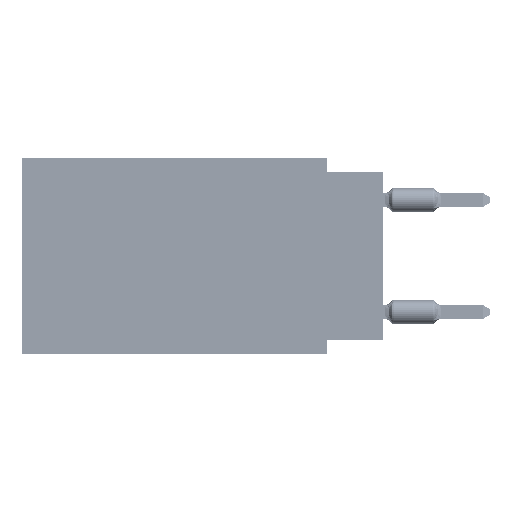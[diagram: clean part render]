
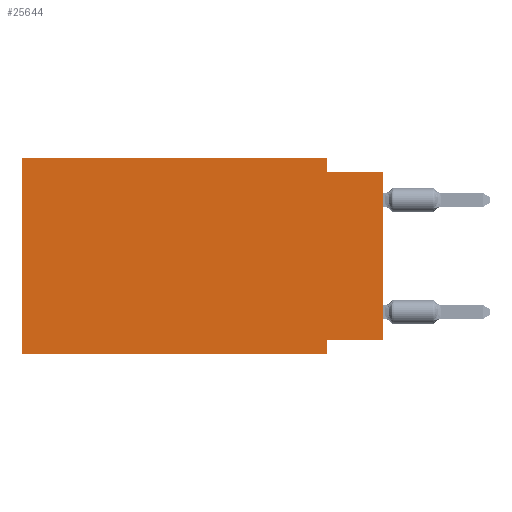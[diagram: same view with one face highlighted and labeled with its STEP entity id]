
A CAD part, left-side view. The second image highlights one B-rep face of the part: STEP entity #25644.
In plain terms, the highlighted planar face has unit normal (-1, 0, 0).
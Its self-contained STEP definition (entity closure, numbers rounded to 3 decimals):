
#2903 = AXIS2_PLACEMENT_3D ( 'NONE', #25191, #89665, #39672 ) ;
#4005 = CARTESIAN_POINT ( 'NONE',  ( 0., 0., -0.635 ) ) ;
#4945 = CARTESIAN_POINT ( 'NONE',  ( 0., 0., 0. ) ) ;
#7699 = CARTESIAN_POINT ( 'NONE',  ( 0., 2.54, -0.635 ) ) ;
#8416 = DIRECTION ( 'NONE',  ( 0., -1., 0. ) ) ;
#8922 = CARTESIAN_POINT ( 'NONE',  ( 0., 16.383, -8.89 ) ) ;
#10558 = VERTEX_POINT ( 'NONE', #29692 ) ;
#10713 = FACE_OUTER_BOUND ( 'NONE', #48097, .T. ) ;
#14119 = VERTEX_POINT ( 'NONE', #87264 ) ;
#14963 = LINE ( 'NONE', #59749, #63827 ) ;
#16705 = ORIENTED_EDGE ( 'NONE', *, *, #35602, .F. ) ;
#18599 = ORIENTED_EDGE ( 'NONE', *, *, #50139, .F. ) ;
#19564 = DIRECTION ( 'NONE',  ( 0., 0., 1. ) ) ;
#20026 = CARTESIAN_POINT ( 'NONE',  ( 0., 16.383, 0. ) ) ;
#20128 = VECTOR ( 'NONE', #69852, 1000. ) ;
#20346 = LINE ( 'NONE', #4005, #20128 ) ;
#20501 = EDGE_CURVE ( 'NONE', #47222, #37222, #57631, .T. ) ;
#20869 = VECTOR ( 'NONE', #86489, 1000. ) ;
#22082 = EDGE_CURVE ( 'NONE', #10558, #37222, #43518, .T. ) ;
#22592 = DIRECTION ( 'NONE',  ( 0., 0., -1. ) ) ;
#25191 = CARTESIAN_POINT ( 'NONE',  ( 0., 16.383, 0. ) ) ;
#25644 = ADVANCED_FACE ( 'NONE', ( #10713 ), #89194, .F. ) ;
#27021 = LINE ( 'NONE', #20026, #58323 ) ;
#28350 = ORIENTED_EDGE ( 'NONE', *, *, #22082, .T. ) ;
#28411 = ORIENTED_EDGE ( 'NONE', *, *, #61844, .T. ) ;
#28534 = VECTOR ( 'NONE', #33438, 1000. ) ;
#29692 = CARTESIAN_POINT ( 'NONE',  ( 0., 16.383, -8.89 ) ) ;
#30540 = LINE ( 'NONE', #59047, #42568 ) ;
#31368 = CARTESIAN_POINT ( 'NONE',  ( 0., 16.383, 0. ) ) ;
#32716 = ORIENTED_EDGE ( 'NONE', *, *, #20501, .F. ) ;
#33438 = DIRECTION ( 'NONE',  ( 0., 0., 1. ) ) ;
#35602 = EDGE_CURVE ( 'NONE', #63766, #37459, #14963, .T. ) ;
#37222 = VERTEX_POINT ( 'NONE', #68739 ) ;
#37440 = ORIENTED_EDGE ( 'NONE', *, *, #44480, .F. ) ;
#37459 = VERTEX_POINT ( 'NONE', #82539 ) ;
#38574 = ORIENTED_EDGE ( 'NONE', *, *, #50134, .F. ) ;
#39672 = DIRECTION ( 'NONE',  ( 0., 0., -1. ) ) ;
#42568 = VECTOR ( 'NONE', #52934, 1000. ) ;
#43086 = VECTOR ( 'NONE', #22592, 1000. ) ;
#43518 = LINE ( 'NONE', #8922, #20869 ) ;
#44480 = EDGE_CURVE ( 'NONE', #37459, #85617, #30540, .T. ) ;
#47222 = VERTEX_POINT ( 'NONE', #86157 ) ;
#48097 = EDGE_LOOP ( 'NONE', ( #28411, #70766, #37440, #16705, #18599, #28350, #32716, #38574 ) ) ;
#48511 = CARTESIAN_POINT ( 'NONE',  ( 0., 0., -8.255 ) ) ;
#50134 = EDGE_CURVE ( 'NONE', #14119, #47222, #76094, .T. ) ;
#50139 = EDGE_CURVE ( 'NONE', #10558, #63766, #27021, .T. ) ;
#50622 = CARTESIAN_POINT ( 'NONE',  ( 0., 2.54, -8.89 ) ) ;
#50859 = VECTOR ( 'NONE', #77950, 1000. ) ;
#52934 = DIRECTION ( 'NONE',  ( 0., 0., -1. ) ) ;
#53810 = EDGE_CURVE ( 'NONE', #85617, #55611, #20346, .T. ) ;
#55611 = VERTEX_POINT ( 'NONE', #64595 ) ;
#57631 = LINE ( 'NONE', #50622, #43086 ) ;
#58323 = VECTOR ( 'NONE', #19564, 1000. ) ;
#59047 = CARTESIAN_POINT ( 'NONE',  ( 0., 2.54, 0. ) ) ;
#59749 = CARTESIAN_POINT ( 'NONE',  ( 0., 16.383, 0. ) ) ;
#61844 = EDGE_CURVE ( 'NONE', #14119, #55611, #82958, .T. ) ;
#63766 = VERTEX_POINT ( 'NONE', #31368 ) ;
#63827 = VECTOR ( 'NONE', #8416, 1000. ) ;
#64595 = CARTESIAN_POINT ( 'NONE',  ( 0., 0., -0.635 ) ) ;
#68739 = CARTESIAN_POINT ( 'NONE',  ( 0., 2.54, -8.89 ) ) ;
#69852 = DIRECTION ( 'NONE',  ( 0., -1., 0. ) ) ;
#70766 = ORIENTED_EDGE ( 'NONE', *, *, #53810, .F. ) ;
#76094 = LINE ( 'NONE', #48511, #50859 ) ;
#77950 = DIRECTION ( 'NONE',  ( 0., 1., 0. ) ) ;
#82539 = CARTESIAN_POINT ( 'NONE',  ( 0., 2.54, 0. ) ) ;
#82958 = LINE ( 'NONE', #4945, #28534 ) ;
#85617 = VERTEX_POINT ( 'NONE', #7699 ) ;
#86157 = CARTESIAN_POINT ( 'NONE',  ( 0., 2.54, -8.255 ) ) ;
#86489 = DIRECTION ( 'NONE',  ( 0., -1., 0. ) ) ;
#87264 = CARTESIAN_POINT ( 'NONE',  ( 0., 0., -8.255 ) ) ;
#89194 = PLANE ( 'NONE',  #2903 ) ;
#89665 = DIRECTION ( 'NONE',  ( 1., 0., 0. ) ) ;
